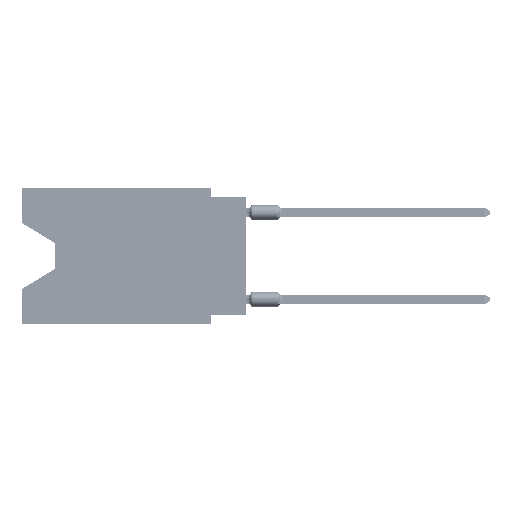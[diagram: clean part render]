
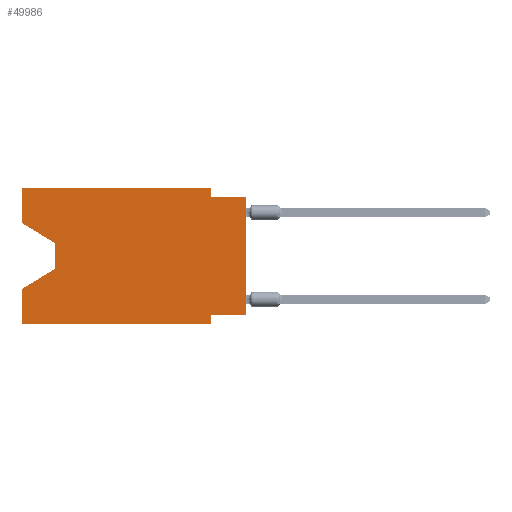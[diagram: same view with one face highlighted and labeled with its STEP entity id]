
A CAD part, left-side view. The second image highlights one B-rep face of the part: STEP entity #49986.
In plain terms, the highlighted planar face has unit normal (-1, 0, 0).
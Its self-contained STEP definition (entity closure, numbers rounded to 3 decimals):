
#664 = CARTESIAN_POINT ( 'NONE',  ( 0., 2.54, 0. ) ) ;
#1852 = VECTOR ( 'NONE', #47124, 1000. ) ;
#2779 = VERTEX_POINT ( 'NONE', #33171 ) ;
#3238 = CARTESIAN_POINT ( 'NONE',  ( 0., 16.383, 0. ) ) ;
#3554 = DIRECTION ( 'NONE',  ( 0., 0., 1. ) ) ;
#6093 = LINE ( 'NONE', #46508, #47285 ) ;
#6477 = CARTESIAN_POINT ( 'NONE',  ( 0., 2.54, -9.906 ) ) ;
#8099 = EDGE_CURVE ( 'NONE', #68196, #56557, #9368, .T. ) ;
#9241 = CARTESIAN_POINT ( 'NONE',  ( 0., 0., 0. ) ) ;
#9368 = LINE ( 'NONE', #26309, #60987 ) ;
#10512 = EDGE_CURVE ( 'NONE', #59573, #64300, #44786, .T. ) ;
#12628 = ORIENTED_EDGE ( 'NONE', *, *, #35480, .F. ) ;
#13178 = ORIENTED_EDGE ( 'NONE', *, *, #55129, .T. ) ;
#13218 = CARTESIAN_POINT ( 'NONE',  ( 0., 16.383, -2.546 ) ) ;
#13642 = DIRECTION ( 'NONE',  ( 0., -1., 0. ) ) ;
#14291 = CARTESIAN_POINT ( 'NONE',  ( 0., 16.383, -2.546 ) ) ;
#14481 = CARTESIAN_POINT ( 'NONE',  ( 0., 16.383, 0. ) ) ;
#15020 = LINE ( 'NONE', #9241, #63486 ) ;
#18292 = EDGE_CURVE ( 'NONE', #44182, #64300, #62409, .T. ) ;
#19543 = EDGE_CURVE ( 'NONE', #31082, #45426, #32802, .T. ) ;
#19856 = PLANE ( 'NONE',  #62111 ) ;
#19903 = VERTEX_POINT ( 'NONE', #49007 ) ;
#22444 = CARTESIAN_POINT ( 'NONE',  ( 0., 16.383, 0. ) ) ;
#23804 = ORIENTED_EDGE ( 'NONE', *, *, #18292, .T. ) ;
#24272 = VECTOR ( 'NONE', #64593, 1000. ) ;
#25524 = VECTOR ( 'NONE', #3554, 1000. ) ;
#25545 = CARTESIAN_POINT ( 'NONE',  ( 0., 0., -9.271 ) ) ;
#25878 = DIRECTION ( 'NONE',  ( 0., 0.855, -0.519 ) ) ;
#26309 = CARTESIAN_POINT ( 'NONE',  ( 0., 2.54, 0. ) ) ;
#31082 = VERTEX_POINT ( 'NONE', #14291 ) ;
#31738 = LINE ( 'NONE', #3238, #45087 ) ;
#31747 = CARTESIAN_POINT ( 'NONE',  ( 0., 13.97, -4.013 ) ) ;
#32401 = CARTESIAN_POINT ( 'NONE',  ( 0., 13.97, -5.893 ) ) ;
#32802 = LINE ( 'NONE', #56282, #25524 ) ;
#32926 = CARTESIAN_POINT ( 'NONE',  ( 0., 13.97, -4.013 ) ) ;
#33171 = CARTESIAN_POINT ( 'NONE',  ( 0., 0., -0.635 ) ) ;
#33299 = DIRECTION ( 'NONE',  ( 0., 0., -1. ) ) ;
#34178 = EDGE_CURVE ( 'NONE', #45426, #68196, #31738, .T. ) ;
#34800 = ORIENTED_EDGE ( 'NONE', *, *, #69817, .T. ) ;
#35246 = VECTOR ( 'NONE', #25878, 1000. ) ;
#35480 = EDGE_CURVE ( 'NONE', #62050, #74536, #6093, .T. ) ;
#35567 = ORIENTED_EDGE ( 'NONE', *, *, #34178, .F. ) ;
#36151 = CARTESIAN_POINT ( 'NONE',  ( 0., 13.97, -5.893 ) ) ;
#37053 = CARTESIAN_POINT ( 'NONE',  ( 0., 16.383, -9.906 ) ) ;
#37959 = DIRECTION ( 'NONE',  ( 1., 0., 0. ) ) ;
#38627 = DIRECTION ( 'NONE',  ( 0., 0., 1. ) ) ;
#38886 = ORIENTED_EDGE ( 'NONE', *, *, #52148, .F. ) ;
#40208 = DIRECTION ( 'NONE',  ( 0., -1., 0. ) ) ;
#40671 = ORIENTED_EDGE ( 'NONE', *, *, #8099, .F. ) ;
#41585 = VECTOR ( 'NONE', #40208, 1000. ) ;
#43091 = ORIENTED_EDGE ( 'NONE', *, *, #10512, .F. ) ;
#44182 = VERTEX_POINT ( 'NONE', #36151 ) ;
#44786 = LINE ( 'NONE', #22444, #51422 ) ;
#45087 = VECTOR ( 'NONE', #13642, 1000. ) ;
#45426 = VERTEX_POINT ( 'NONE', #57476 ) ;
#45834 = EDGE_LOOP ( 'NONE', ( #72790, #13178, #23804, #43091, #34800, #38886, #12628, #65107, #64676, #40671, #35567, #47778 ) ) ;
#46508 = CARTESIAN_POINT ( 'NONE',  ( 0., 0., -9.271 ) ) ;
#46801 = VECTOR ( 'NONE', #59107, 1000. ) ;
#47124 = DIRECTION ( 'NONE',  ( 0., -0.855, -0.519 ) ) ;
#47285 = VECTOR ( 'NONE', #71103, 1000. ) ;
#47778 = ORIENTED_EDGE ( 'NONE', *, *, #19543, .F. ) ;
#49007 = CARTESIAN_POINT ( 'NONE',  ( 0., 2.54, -9.906 ) ) ;
#49986 = ADVANCED_FACE ( 'NONE', ( #73721 ), #19856, .F. ) ;
#50624 = CARTESIAN_POINT ( 'NONE',  ( 0., 0., -0.635 ) ) ;
#50904 = DIRECTION ( 'NONE',  ( 0., 0., -1. ) ) ;
#50916 = CARTESIAN_POINT ( 'NONE',  ( 0., 2.54, -0.635 ) ) ;
#51422 = VECTOR ( 'NONE', #38627, 1000. ) ;
#52148 = EDGE_CURVE ( 'NONE', #74536, #19903, #59206, .T. ) ;
#52897 = LINE ( 'NONE', #13218, #1852 ) ;
#55129 = EDGE_CURVE ( 'NONE', #70001, #44182, #73319, .T. ) ;
#55301 = VECTOR ( 'NONE', #33299, 1000. ) ;
#56282 = CARTESIAN_POINT ( 'NONE',  ( 0., 16.383, 0. ) ) ;
#56557 = VERTEX_POINT ( 'NONE', #50916 ) ;
#56835 = CARTESIAN_POINT ( 'NONE',  ( 0., 16.383, -7.36 ) ) ;
#57476 = CARTESIAN_POINT ( 'NONE',  ( 0., 16.383, 0. ) ) ;
#59107 = DIRECTION ( 'NONE',  ( 0., -1., 0. ) ) ;
#59206 = LINE ( 'NONE', #6477, #24272 ) ;
#59573 = VERTEX_POINT ( 'NONE', #37053 ) ;
#60987 = VECTOR ( 'NONE', #50904, 1000. ) ;
#61873 = EDGE_CURVE ( 'NONE', #31082, #70001, #52897, .T. ) ;
#62050 = VERTEX_POINT ( 'NONE', #25545 ) ;
#62111 = AXIS2_PLACEMENT_3D ( 'NONE', #14481, #37959, #75221 ) ;
#62409 = LINE ( 'NONE', #32401, #35246 ) ;
#63486 = VECTOR ( 'NONE', #73507, 1000. ) ;
#63728 = CARTESIAN_POINT ( 'NONE',  ( 0., 2.54, -9.271 ) ) ;
#64300 = VERTEX_POINT ( 'NONE', #56835 ) ;
#64488 = LINE ( 'NONE', #64882, #46801 ) ;
#64593 = DIRECTION ( 'NONE',  ( 0., 0., -1. ) ) ;
#64676 = ORIENTED_EDGE ( 'NONE', *, *, #67193, .F. ) ;
#64882 = CARTESIAN_POINT ( 'NONE',  ( 0., 16.383, -9.906 ) ) ;
#64948 = EDGE_CURVE ( 'NONE', #62050, #2779, #15020, .T. ) ;
#65107 = ORIENTED_EDGE ( 'NONE', *, *, #64948, .T. ) ;
#67193 = EDGE_CURVE ( 'NONE', #56557, #2779, #69439, .T. ) ;
#68196 = VERTEX_POINT ( 'NONE', #664 ) ;
#69439 = LINE ( 'NONE', #50624, #41585 ) ;
#69817 = EDGE_CURVE ( 'NONE', #59573, #19903, #64488, .T. ) ;
#70001 = VERTEX_POINT ( 'NONE', #31747 ) ;
#71103 = DIRECTION ( 'NONE',  ( 0., 1., 0. ) ) ;
#72790 = ORIENTED_EDGE ( 'NONE', *, *, #61873, .T. ) ;
#73319 = LINE ( 'NONE', #32926, #55301 ) ;
#73507 = DIRECTION ( 'NONE',  ( 0., 0., 1. ) ) ;
#73721 = FACE_OUTER_BOUND ( 'NONE', #45834, .T. ) ;
#74536 = VERTEX_POINT ( 'NONE', #63728 ) ;
#75221 = DIRECTION ( 'NONE',  ( 0., 0., -1. ) ) ;
